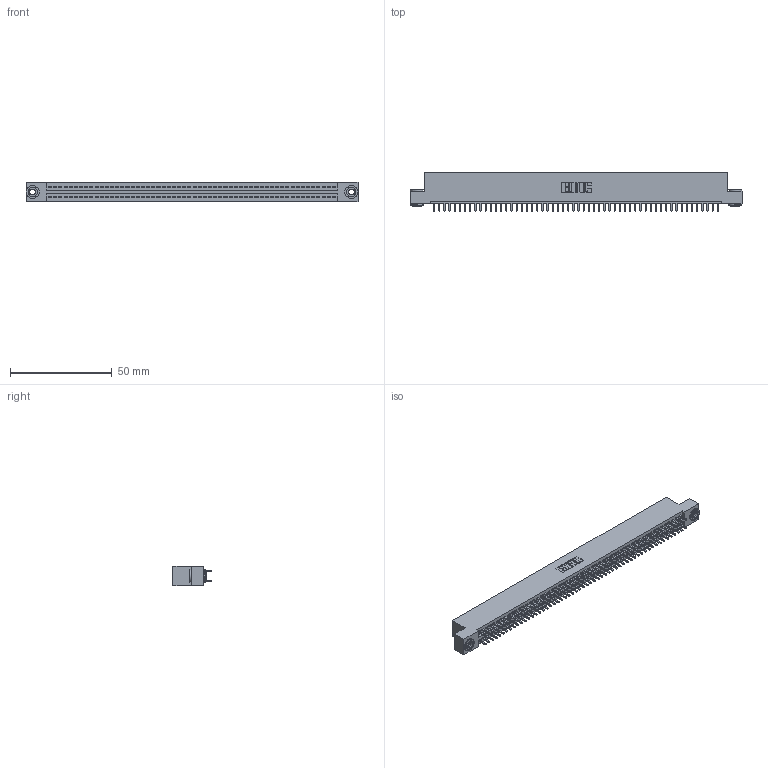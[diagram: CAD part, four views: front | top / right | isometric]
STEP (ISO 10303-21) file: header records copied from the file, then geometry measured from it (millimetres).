
FILE_DESCRIPTION (( 'STEP AP203' ), '1' );
FILE_NAME ('345-112-521-203.STEP', '2018-10-07T13:48:23', ( '' ), ( '' ), 'SwSTEP 2.0', 'SolidWorks 2016', '' );
FILE_SCHEMA (( 'CONFIG_CONTROL_DESIGN' ));
Length unit declared in the file: inch
Products named in the file (4): 345-292-001_345-293-121; 345-112-521-203; 345 Part_Flush Mounting Lugs - 0.156 Dia-TH; 345-250-002_345-250-002-102
Assembly tree (115 placements, depth 2):
  345-112-521-203
    345 Part_Flush Mounting Lugs - 0.156 Dia-TH
    345-292-001_345-293-121  x112
    345-250-002_345-250-002-102  x2
Bounding box: 163.45 x 18.72 x 9.4 mm (x, y, z)
Volume: 15981.2 mm3; surface area: 23801.5 mm2
Topology: 115 solids, 115 shells, 5764 faces, 17105 edges, 11250 vertices
Faces by surface type: plane 3786, cylinder 1970, cone 8
Entity records: 42722 total; most frequent: CARTESIAN_POINT 7123, ORIENTED_EDGE 7050, DIRECTION 6295, EDGE_CURVE 3525, LINE 3145, VECTOR 3145, VERTEX_POINT 2346, AXIS2_PLACEMENT_3D 1575
